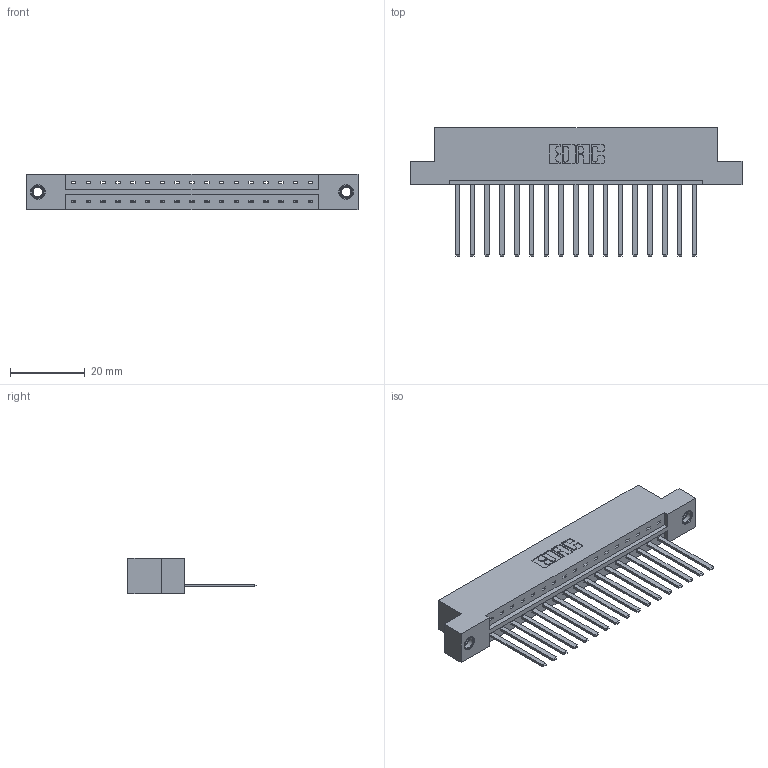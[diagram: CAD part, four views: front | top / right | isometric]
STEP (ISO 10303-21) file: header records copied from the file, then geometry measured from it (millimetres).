
FILE_DESCRIPTION (( 'STEP AP203' ), '1' );
FILE_NAME ('833-017-544-107.STEP', '2020-05-31T20:23:32', ( '' ), ( '' ), 'SwSTEP 2.0', 'SolidWorks 2020', '' );
FILE_SCHEMA (( 'CONFIG_CONTROL_DESIGN' ));
Length unit declared in the file: inch
Products named in the file (4): 345-250-001_345-250-005-103; 833-017-544-107; 345-292-001_345-293-144; 833 Part_Flush - .156 Dia - TI
Assembly tree (20 placements, depth 2):
  833-017-544-107
    833 Part_Flush - .156 Dia - TI
    345-292-001_345-293-144  x17
    345-250-001_345-250-005-103  x2
Bounding box: 88.9 x 34.3 x 9.4 mm (x, y, z)
Volume: 8914.2 mm3; surface area: 10159.1 mm2
Topology: 20 solids, 20 shells, 1058 faces, 3133 edges, 2058 vertices
Faces by surface type: plane 748, cylinder 294, cone 12, torus 4
Entity records: 14628 total; most frequent: CARTESIAN_POINT 2508, ORIENTED_EDGE 2454, DIRECTION 2195, EDGE_CURVE 1227, LINE 1083, VECTOR 1083, VERTEX_POINT 812, AXIS2_PLACEMENT_3D 556
